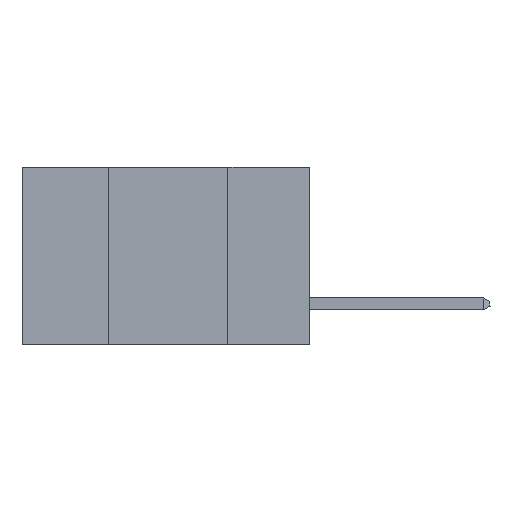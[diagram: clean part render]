
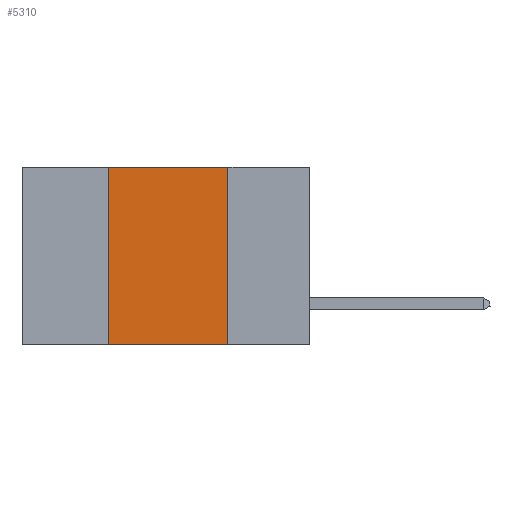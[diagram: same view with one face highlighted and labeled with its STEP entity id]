
A CAD part, left-side view. The second image highlights one B-rep face of the part: STEP entity #5310.
In plain terms, the highlighted planar face has unit normal (-1, 0, 0).
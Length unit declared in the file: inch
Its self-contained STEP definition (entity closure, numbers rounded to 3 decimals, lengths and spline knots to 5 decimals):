
#608 = VERTEX_POINT ( 'NONE', #17249 ) ;
#1308 = EDGE_LOOP ( 'NONE', ( #10881, #28442, #15049, #36257 ) ) ;
#2671 = CARTESIAN_POINT ( 'NONE',  ( 0., 0.6, -0.37 ) ) ;
#2821 = AXIS2_PLACEMENT_3D ( 'NONE', #28679, #32585, #35794 ) ;
#4730 = CARTESIAN_POINT ( 'NONE',  ( 0., 0.17, 0. ) ) ;
#5310 = ADVANCED_FACE ( 'NONE', ( #36686 ), #24522, .F. ) ;
#6076 = LINE ( 'NONE', #30234, #17933 ) ;
#10747 = LINE ( 'NONE', #4730, #19916 ) ;
#10881 = ORIENTED_EDGE ( 'NONE', *, *, #17133, .F. ) ;
#11391 = VERTEX_POINT ( 'NONE', #16351 ) ;
#11597 = VERTEX_POINT ( 'NONE', #26818 ) ;
#11892 = CARTESIAN_POINT ( 'NONE',  ( 0., 0.6, 0. ) ) ;
#15049 = ORIENTED_EDGE ( 'NONE', *, *, #40607, .F. ) ;
#15506 = VECTOR ( 'NONE', #40098, 39.37008 ) ;
#16351 = CARTESIAN_POINT ( 'NONE',  ( 0., 0.42, 0. ) ) ;
#17133 = EDGE_CURVE ( 'NONE', #608, #11597, #10747, .T. ) ;
#17249 = CARTESIAN_POINT ( 'NONE',  ( 0., 0.17, 0. ) ) ;
#17933 = VECTOR ( 'NONE', #20171, 39.37008 ) ;
#19916 = VECTOR ( 'NONE', #25507, 39.37008 ) ;
#20171 = DIRECTION ( 'NONE',  ( 0., 0., 1. ) ) ;
#21297 = VERTEX_POINT ( 'NONE', #33426 ) ;
#21343 = EDGE_CURVE ( 'NONE', #21297, #11597, #35356, .T. ) ;
#24522 = PLANE ( 'NONE',  #2821 ) ;
#25507 = DIRECTION ( 'NONE',  ( 0., 0., -1. ) ) ;
#26818 = CARTESIAN_POINT ( 'NONE',  ( 0., 0.17, -0.37 ) ) ;
#28442 = ORIENTED_EDGE ( 'NONE', *, *, #28869, .F. ) ;
#28679 = CARTESIAN_POINT ( 'NONE',  ( 0., 0.6, 0. ) ) ;
#28869 = EDGE_CURVE ( 'NONE', #11391, #608, #39754, .T. ) ;
#30234 = CARTESIAN_POINT ( 'NONE',  ( 0., 0.42, 0. ) ) ;
#30573 = VECTOR ( 'NONE', #39044, 39.37008 ) ;
#32585 = DIRECTION ( 'NONE',  ( 1., 0., 0. ) ) ;
#33426 = CARTESIAN_POINT ( 'NONE',  ( 0., 0.42, -0.37 ) ) ;
#35356 = LINE ( 'NONE', #2671, #15506 ) ;
#35794 = DIRECTION ( 'NONE',  ( 0., 0., -1. ) ) ;
#36257 = ORIENTED_EDGE ( 'NONE', *, *, #21343, .T. ) ;
#36686 = FACE_OUTER_BOUND ( 'NONE', #1308, .T. ) ;
#39044 = DIRECTION ( 'NONE',  ( 0., -1., 0. ) ) ;
#39754 = LINE ( 'NONE', #11892, #30573 ) ;
#40098 = DIRECTION ( 'NONE',  ( 0., -1., 0. ) ) ;
#40607 = EDGE_CURVE ( 'NONE', #21297, #11391, #6076, .T. ) ;
